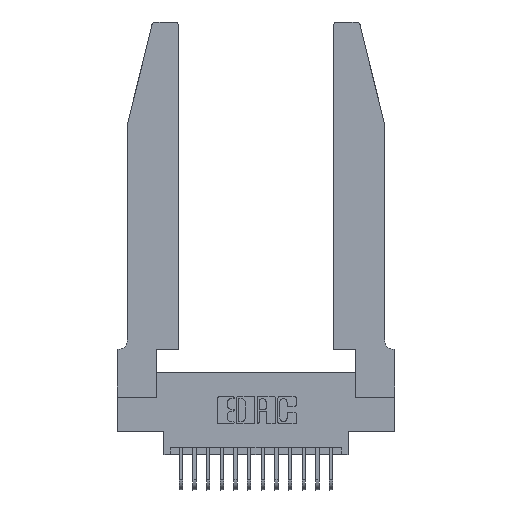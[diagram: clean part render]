
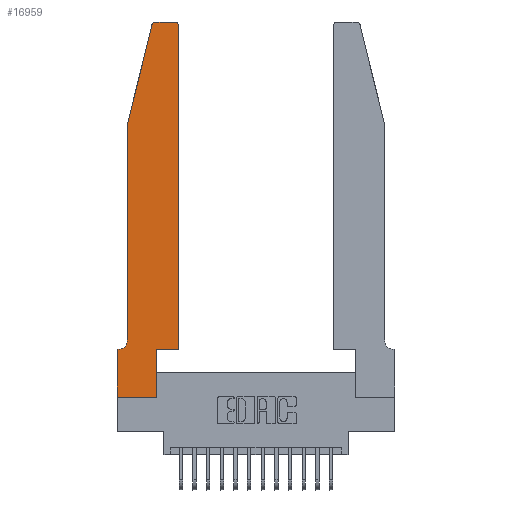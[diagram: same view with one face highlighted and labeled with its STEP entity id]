
A CAD part, top view. The second image highlights one B-rep face of the part: STEP entity #16959.
In plain terms, the highlighted planar face has unit normal (0, 0, 1).
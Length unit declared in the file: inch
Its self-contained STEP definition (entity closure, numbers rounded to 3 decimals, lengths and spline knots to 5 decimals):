
#272 = EDGE_CURVE ( 'NONE', #6562, #4828, #16026, .T. ) ;
#419 = ORIENTED_EDGE ( 'NONE', *, *, #13749, .T. ) ;
#608 = DIRECTION ( 'NONE',  ( 0., 0., 1. ) ) ;
#624 = EDGE_CURVE ( 'NONE', #1542, #2079, #14816, .T. ) ;
#671 = ORIENTED_EDGE ( 'NONE', *, *, #3072, .T. ) ;
#1542 = VERTEX_POINT ( 'NONE', #1888 ) ;
#1671 = LINE ( 'NONE', #13905, #9481 ) ;
#1778 = CARTESIAN_POINT ( 'NONE',  ( 0.0055, 0.42, 0.37 ) ) ;
#1888 = CARTESIAN_POINT ( 'NONE',  ( 0.4505, 0.35, 0.37 ) ) ;
#2039 = DIRECTION ( 'NONE',  ( -0.239, -0.971, 0. ) ) ;
#2079 = VERTEX_POINT ( 'NONE', #15655 ) ;
#2249 = CARTESIAN_POINT ( 'NONE',  ( 0.0755, 0.35, 0.37 ) ) ;
#2508 = AXIS2_PLACEMENT_3D ( 'NONE', #1778, #12644, #3309 ) ;
#2537 = CARTESIAN_POINT ( 'NONE',  ( 0.2865, 0.35, 0.37 ) ) ;
#2632 = ORIENTED_EDGE ( 'NONE', *, *, #272, .T. ) ;
#3072 = EDGE_CURVE ( 'NONE', #3469, #6562, #1671, .T. ) ;
#3305 = CARTESIAN_POINT ( 'NONE',  ( 0.0755, 2., 0.37 ) ) ;
#3309 = DIRECTION ( 'NONE',  ( -1., 0., 0. ) ) ;
#3346 = ORIENTED_EDGE ( 'NONE', *, *, #18007, .T. ) ;
#3422 = EDGE_CURVE ( 'NONE', #9387, #1542, #3554, .T. ) ;
#3469 = VERTEX_POINT ( 'NONE', #5545 ) ;
#3554 = LINE ( 'NONE', #13216, #19486 ) ;
#3591 = ORIENTED_EDGE ( 'NONE', *, *, #3422, .T. ) ;
#4073 = ORIENTED_EDGE ( 'NONE', *, *, #624, .T. ) ;
#4312 = ORIENTED_EDGE ( 'NONE', *, *, #12559, .T. ) ;
#4383 = VECTOR ( 'NONE', #12019, 39.37008 ) ;
#4395 = CARTESIAN_POINT ( 'NONE',  ( 0.0755, 2., 0.37 ) ) ;
#4606 = AXIS2_PLACEMENT_3D ( 'NONE', #4638, #15485, #6232 ) ;
#4638 = CARTESIAN_POINT ( 'NONE',  ( 0.4205, 2.72, 0.37 ) ) ;
#4718 = DIRECTION ( 'NONE',  ( 0., 0., 1. ) ) ;
#4825 = CARTESIAN_POINT ( 'NONE',  ( 0.0755, 0.42, 0.37 ) ) ;
#4828 = VERTEX_POINT ( 'NONE', #13857 ) ;
#4870 = DIRECTION ( 'NONE',  ( 0., -1., 0. ) ) ;
#5545 = CARTESIAN_POINT ( 'NONE',  ( 0., 0.35, 0.37 ) ) ;
#6055 = ORIENTED_EDGE ( 'NONE', *, *, #10556, .T. ) ;
#6163 = EDGE_CURVE ( 'NONE', #12516, #18027, #6969, .T. ) ;
#6232 = DIRECTION ( 'NONE',  ( 1., 0., 0. ) ) ;
#6562 = VERTEX_POINT ( 'NONE', #8864 ) ;
#6969 = CIRCLE ( 'NONE', #11720, 0.03 ) ;
#6992 = CIRCLE ( 'NONE', #4606, 0.03 ) ;
#7608 = LINE ( 'NONE', #11386, #15781 ) ;
#7670 = VERTEX_POINT ( 'NONE', #10307 ) ;
#7867 = VECTOR ( 'NONE', #18615, 39.37008 ) ;
#8029 = ORIENTED_EDGE ( 'NONE', *, *, #11179, .T. ) ;
#8316 = CARTESIAN_POINT ( 'NONE',  ( 0.2605, 2.75, 0.37 ) ) ;
#8427 = PLANE ( 'NONE',  #14278 ) ;
#8864 = CARTESIAN_POINT ( 'NONE',  ( 0., 0., 0.37 ) ) ;
#9209 = LINE ( 'NONE', #3305, #16870 ) ;
#9387 = VERTEX_POINT ( 'NONE', #2537 ) ;
#9481 = VECTOR ( 'NONE', #12425, 39.37008 ) ;
#10045 = DIRECTION ( 'NONE',  ( -1., 0., 0. ) ) ;
#10197 = VERTEX_POINT ( 'NONE', #4395 ) ;
#10307 = CARTESIAN_POINT ( 'NONE',  ( 0.0055, 0.35, 0.37 ) ) ;
#10460 = CARTESIAN_POINT ( 'NONE',  ( 0.2865, 0.35, 0.37 ) ) ;
#10556 = EDGE_CURVE ( 'NONE', #16651, #12516, #11726, .T. ) ;
#11179 = EDGE_CURVE ( 'NONE', #16145, #7670, #14116, .T. ) ;
#11188 = CARTESIAN_POINT ( 'NONE',  ( 0.25487, 2.72718, 0.37 ) ) ;
#11292 = EDGE_CURVE ( 'NONE', #18027, #10197, #7608, .T. ) ;
#11365 = CARTESIAN_POINT ( 'NONE',  ( 0.4505, 0.35, 0.37 ) ) ;
#11386 = CARTESIAN_POINT ( 'NONE',  ( 0.0755, 2., 0.37 ) ) ;
#11444 = ORIENTED_EDGE ( 'NONE', *, *, #17146, .T. ) ;
#11549 = DIRECTION ( 'NONE',  ( 1., 0., 0. ) ) ;
#11720 = AXIS2_PLACEMENT_3D ( 'NONE', #14041, #4718, #15562 ) ;
#11726 = LINE ( 'NONE', #8316, #15296 ) ;
#12019 = DIRECTION ( 'NONE',  ( 0., 1., 0. ) ) ;
#12425 = DIRECTION ( 'NONE',  ( 0., -1., 0. ) ) ;
#12516 = VERTEX_POINT ( 'NONE', #16122 ) ;
#12559 = EDGE_CURVE ( 'NONE', #7670, #3469, #14540, .T. ) ;
#12644 = DIRECTION ( 'NONE',  ( 0., 0., -1. ) ) ;
#13216 = CARTESIAN_POINT ( 'NONE',  ( 0.4505, 0.35, 0.37 ) ) ;
#13749 = EDGE_CURVE ( 'NONE', #2079, #16651, #6992, .T. ) ;
#13857 = CARTESIAN_POINT ( 'NONE',  ( 0.2865, 0., 0.37 ) ) ;
#13905 = CARTESIAN_POINT ( 'NONE',  ( 0., 0., 0.37 ) ) ;
#14041 = CARTESIAN_POINT ( 'NONE',  ( 0.284, 2.72, 0.37 ) ) ;
#14063 = VECTOR ( 'NONE', #10045, 39.37008 ) ;
#14116 = CIRCLE ( 'NONE', #2508, 0.07 ) ;
#14278 = AXIS2_PLACEMENT_3D ( 'NONE', #19123, #608, #11549 ) ;
#14281 = ORIENTED_EDGE ( 'NONE', *, *, #6163, .T. ) ;
#14342 = VECTOR ( 'NONE', #15534, 39.37008 ) ;
#14540 = LINE ( 'NONE', #2249, #14063 ) ;
#14734 = DIRECTION ( 'NONE',  ( 1., 0., 0. ) ) ;
#14752 = ORIENTED_EDGE ( 'NONE', *, *, #11292, .T. ) ;
#14816 = LINE ( 'NONE', #11365, #14342 ) ;
#14872 = EDGE_LOOP ( 'NONE', ( #6055, #14281, #14752, #3346, #8029, #4312, #671, #2632, #11444, #3591, #4073, #419 ) ) ;
#15296 = VECTOR ( 'NONE', #17506, 39.37008 ) ;
#15485 = DIRECTION ( 'NONE',  ( 0., 0., 1. ) ) ;
#15534 = DIRECTION ( 'NONE',  ( 0., 1., 0. ) ) ;
#15562 = DIRECTION ( 'NONE',  ( 1., 0., 0. ) ) ;
#15655 = CARTESIAN_POINT ( 'NONE',  ( 0.4505, 2.72, 0.37 ) ) ;
#15781 = VECTOR ( 'NONE', #2039, 39.37008 ) ;
#16026 = LINE ( 'NONE', #19518, #7867 ) ;
#16122 = CARTESIAN_POINT ( 'NONE',  ( 0.284, 2.75, 0.37 ) ) ;
#16145 = VERTEX_POINT ( 'NONE', #4825 ) ;
#16264 = LINE ( 'NONE', #10460, #4383 ) ;
#16651 = VERTEX_POINT ( 'NONE', #16890 ) ;
#16870 = VECTOR ( 'NONE', #4870, 39.37008 ) ;
#16890 = CARTESIAN_POINT ( 'NONE',  ( 0.4205, 2.75, 0.37 ) ) ;
#16959 = ADVANCED_FACE ( 'NONE', ( #19585 ), #8427, .T. ) ;
#17146 = EDGE_CURVE ( 'NONE', #4828, #9387, #16264, .T. ) ;
#17506 = DIRECTION ( 'NONE',  ( -1., 0., 0. ) ) ;
#18007 = EDGE_CURVE ( 'NONE', #10197, #16145, #9209, .T. ) ;
#18027 = VERTEX_POINT ( 'NONE', #11188 ) ;
#18615 = DIRECTION ( 'NONE',  ( 1., 0., 0. ) ) ;
#19123 = CARTESIAN_POINT ( 'NONE',  ( 0., 0.35, 0.37 ) ) ;
#19486 = VECTOR ( 'NONE', #14734, 39.37008 ) ;
#19518 = CARTESIAN_POINT ( 'NONE',  ( 0., 0., 0.37 ) ) ;
#19585 = FACE_OUTER_BOUND ( 'NONE', #14872, .T. ) ;
